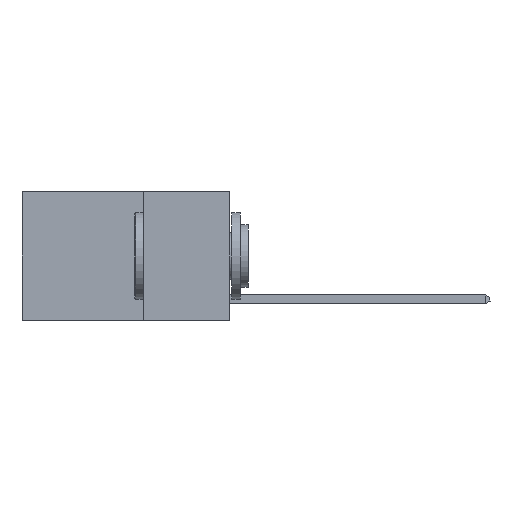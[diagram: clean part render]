
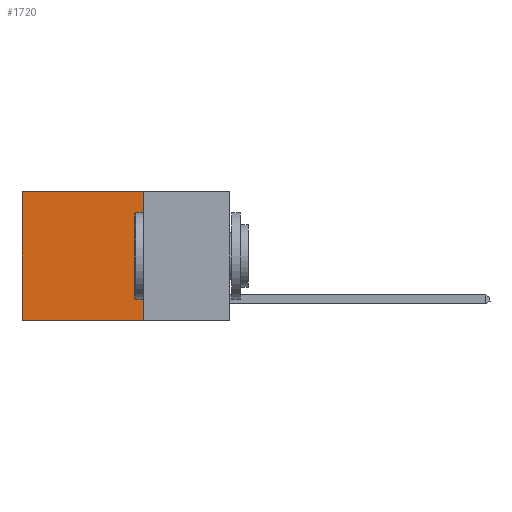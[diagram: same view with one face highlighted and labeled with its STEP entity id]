
A CAD part, left-side view. The second image highlights one B-rep face of the part: STEP entity #1720.
In plain terms, the highlighted planar face has unit normal (-1, 0, 0).
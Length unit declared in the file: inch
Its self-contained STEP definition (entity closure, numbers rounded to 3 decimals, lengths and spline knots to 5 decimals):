
#548 = EDGE_CURVE ( 'NONE', #720, #14955, #20223, .T. ) ;
#720 = VERTEX_POINT ( 'NONE', #7199 ) ;
#1704 = CARTESIAN_POINT ( 'NONE',  ( 0.2625, 0.25, -0.37 ) ) ;
#1720 = ADVANCED_FACE ( 'NONE', ( #17809 ), #9200, .F. ) ;
#3068 = DIRECTION ( 'NONE',  ( 0., 1., 0. ) ) ;
#3610 = CARTESIAN_POINT ( 'NONE',  ( 0.2625, 0.25, -0.37 ) ) ;
#4143 = EDGE_CURVE ( 'NONE', #11233, #14955, #16592, .T. ) ;
#4967 = VECTOR ( 'NONE', #3068, 39.37008 ) ;
#5970 = EDGE_CURVE ( 'NONE', #8512, #720, #13928, .T. ) ;
#7078 = ORIENTED_EDGE ( 'NONE', *, *, #17779, .F. ) ;
#7199 = CARTESIAN_POINT ( 'NONE',  ( 0.2625, 0.6, 0. ) ) ;
#7480 = CARTESIAN_POINT ( 'NONE',  ( 0.2625, 0.25, 0. ) ) ;
#8512 = VERTEX_POINT ( 'NONE', #10458 ) ;
#8516 = CARTESIAN_POINT ( 'NONE',  ( 0.2625, 0.25, 0. ) ) ;
#8638 = DIRECTION ( 'NONE',  ( 0., 0., -1. ) ) ;
#8761 = DIRECTION ( 'NONE',  ( 0., 1., 0. ) ) ;
#9014 = AXIS2_PLACEMENT_3D ( 'NONE', #7480, #14372, #12678 ) ;
#9031 = ORIENTED_EDGE ( 'NONE', *, *, #5970, .T. ) ;
#9200 = PLANE ( 'NONE',  #9014 ) ;
#9229 = ORIENTED_EDGE ( 'NONE', *, *, #4143, .F. ) ;
#9460 = CARTESIAN_POINT ( 'NONE',  ( 0.2625, 0.6, -0.37 ) ) ;
#10335 = CARTESIAN_POINT ( 'NONE',  ( 0.2625, 0.25, 0. ) ) ;
#10458 = CARTESIAN_POINT ( 'NONE',  ( 0.2625, 0.25, 0. ) ) ;
#11233 = VERTEX_POINT ( 'NONE', #3610 ) ;
#12658 = VECTOR ( 'NONE', #8638, 39.37008 ) ;
#12678 = DIRECTION ( 'NONE',  ( 0., 0., -1. ) ) ;
#13493 = ORIENTED_EDGE ( 'NONE', *, *, #548, .T. ) ;
#13928 = LINE ( 'NONE', #10335, #14483 ) ;
#14372 = DIRECTION ( 'NONE',  ( 1., 0., 0. ) ) ;
#14385 = EDGE_LOOP ( 'NONE', ( #13493, #9229, #7078, #9031 ) ) ;
#14483 = VECTOR ( 'NONE', #8761, 39.37008 ) ;
#14955 = VERTEX_POINT ( 'NONE', #9460 ) ;
#15120 = CARTESIAN_POINT ( 'NONE',  ( 0.2625, 0.6, 0. ) ) ;
#16592 = LINE ( 'NONE', #1704, #4967 ) ;
#17545 = LINE ( 'NONE', #8516, #12658 ) ;
#17779 = EDGE_CURVE ( 'NONE', #8512, #11233, #17545, .T. ) ;
#17809 = FACE_OUTER_BOUND ( 'NONE', #14385, .T. ) ;
#18316 = DIRECTION ( 'NONE',  ( 0., 0., -1. ) ) ;
#20223 = LINE ( 'NONE', #15120, #21589 ) ;
#21589 = VECTOR ( 'NONE', #18316, 39.37008 ) ;
